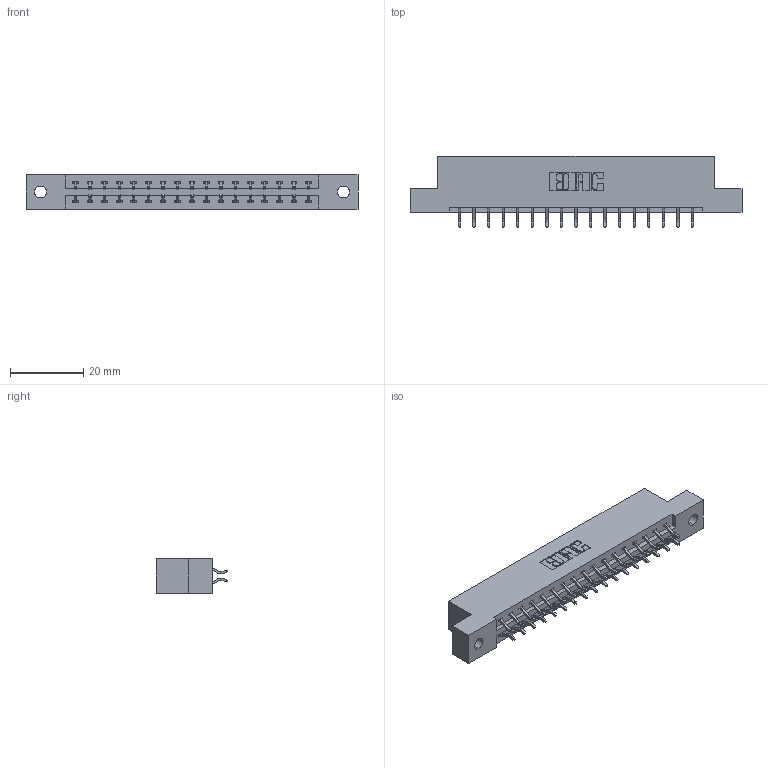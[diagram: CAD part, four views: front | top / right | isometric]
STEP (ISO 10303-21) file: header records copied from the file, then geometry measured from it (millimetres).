
FILE_DESCRIPTION (( 'STEP AP203' ), '1' );
FILE_NAME ('337-034-556-202.STEP', '2019-10-08T20:19:23', ( '' ), ( '' ), 'SwSTEP 2.0', 'SolidWorks 2016', '' );
FILE_SCHEMA (( 'CONFIG_CONTROL_DESIGN' ));
Length unit declared in the file: inch
Products named in the file (3): 345-292-001_556 Tail; 337 Part_Flush Mounting Lugs - 0.128 Dia; 337-034-556-202
Assembly tree (35 placements, depth 2):
  337-034-556-202
    337 Part_Flush Mounting Lugs - 0.128 Dia
    345-292-001_556 Tail  x34
Bounding box: 90.37 x 19.57 x 9.4 mm (x, y, z)
Volume: 9153.4 mm3; surface area: 9796.6 mm2
Topology: 35 solids, 35 shells, 2154 faces, 6397 edges, 4218 vertices
Faces by surface type: plane 1498, cylinder 656
Entity records: 16637 total; most frequent: CARTESIAN_POINT 2838, ORIENTED_EDGE 2762, DIRECTION 2449, EDGE_CURVE 1381, LINE 1245, VECTOR 1245, VERTEX_POINT 918, AXIS2_PLACEMENT_3D 602
